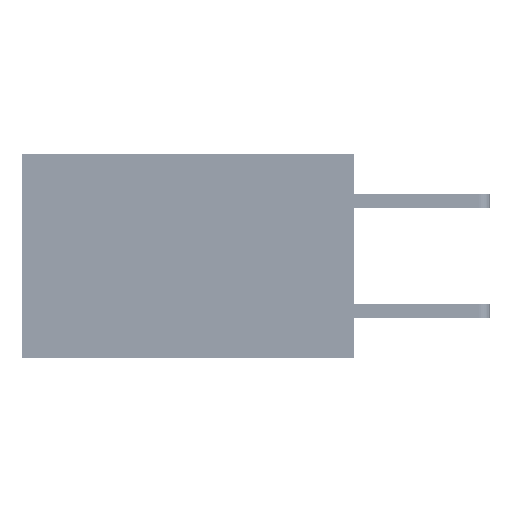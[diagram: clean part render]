
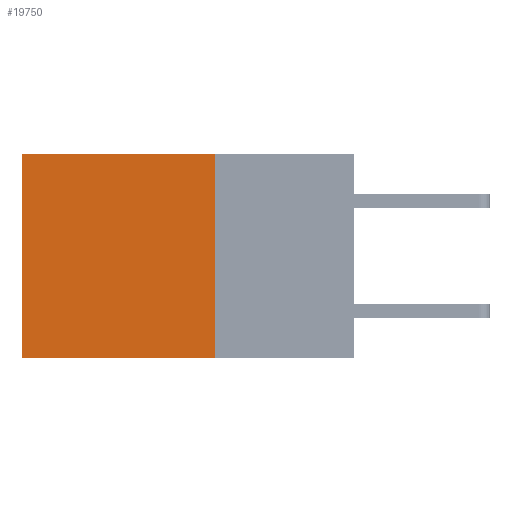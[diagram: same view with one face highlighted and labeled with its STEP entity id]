
A CAD part, left-side view. The second image highlights one B-rep face of the part: STEP entity #19750.
In plain terms, the highlighted planar face has unit normal (-1, 0, 0).
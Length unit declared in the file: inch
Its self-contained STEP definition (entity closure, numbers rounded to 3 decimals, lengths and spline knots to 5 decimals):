
#523 = CARTESIAN_POINT ( 'NONE',  ( 0.2875, 0.25, 0. ) ) ;
#953 = DIRECTION ( 'NONE',  ( 0., 1., 0. ) ) ;
#2493 = FACE_OUTER_BOUND ( 'NONE', #21418, .T. ) ;
#2666 = CARTESIAN_POINT ( 'NONE',  ( 0.2875, 0.25, -0.37 ) ) ;
#4001 = CARTESIAN_POINT ( 'NONE',  ( 0.2875, 0.6, -0.37 ) ) ;
#5000 = EDGE_CURVE ( 'NONE', #21283, #20877, #48073, .T. ) ;
#7228 = DIRECTION ( 'NONE',  ( 0., 0., -1. ) ) ;
#9214 = EDGE_CURVE ( 'NONE', #47405, #21283, #42677, .T. ) ;
#10353 = VECTOR ( 'NONE', #34034, 39.37008 ) ;
#12390 = ORIENTED_EDGE ( 'NONE', *, *, #29195, .T. ) ;
#13457 = LINE ( 'NONE', #523, #33226 ) ;
#13883 = CARTESIAN_POINT ( 'NONE',  ( 0.2875, 0.25, 0. ) ) ;
#17566 = VERTEX_POINT ( 'NONE', #39093 ) ;
#18250 = CARTESIAN_POINT ( 'NONE',  ( 0.2875, 0.6, 0. ) ) ;
#18547 = PLANE ( 'NONE',  #25000 ) ;
#19750 = ADVANCED_FACE ( 'NONE', ( #2493 ), #18547, .F. ) ;
#20877 = VERTEX_POINT ( 'NONE', #4001 ) ;
#21283 = VERTEX_POINT ( 'NONE', #2666 ) ;
#21418 = EDGE_LOOP ( 'NONE', ( #23881, #41360, #47659, #12390 ) ) ;
#23881 = ORIENTED_EDGE ( 'NONE', *, *, #46150, .T. ) ;
#25000 = AXIS2_PLACEMENT_3D ( 'NONE', #46219, #42850, #45731 ) ;
#25775 = LINE ( 'NONE', #18250, #10353 ) ;
#29195 = EDGE_CURVE ( 'NONE', #47405, #17566, #13457, .T. ) ;
#33226 = VECTOR ( 'NONE', #43988, 39.37008 ) ;
#34034 = DIRECTION ( 'NONE',  ( 0., 0., -1. ) ) ;
#34204 = VECTOR ( 'NONE', #7228, 39.37008 ) ;
#36427 = CARTESIAN_POINT ( 'NONE',  ( 0.2875, 0.25, -0.37 ) ) ;
#39093 = CARTESIAN_POINT ( 'NONE',  ( 0.2875, 0.6, 0. ) ) ;
#41360 = ORIENTED_EDGE ( 'NONE', *, *, #5000, .F. ) ;
#42677 = LINE ( 'NONE', #47058, #34204 ) ;
#42850 = DIRECTION ( 'NONE',  ( 1., 0., 0. ) ) ;
#43988 = DIRECTION ( 'NONE',  ( 0., 1., 0. ) ) ;
#45731 = DIRECTION ( 'NONE',  ( 0., 0., -1. ) ) ;
#46150 = EDGE_CURVE ( 'NONE', #17566, #20877, #25775, .T. ) ;
#46219 = CARTESIAN_POINT ( 'NONE',  ( 0.2875, 0.25, 0. ) ) ;
#47058 = CARTESIAN_POINT ( 'NONE',  ( 0.2875, 0.25, 0. ) ) ;
#47405 = VERTEX_POINT ( 'NONE', #13883 ) ;
#47659 = ORIENTED_EDGE ( 'NONE', *, *, #9214, .F. ) ;
#48073 = LINE ( 'NONE', #36427, #49959 ) ;
#49959 = VECTOR ( 'NONE', #953, 39.37008 ) ;
